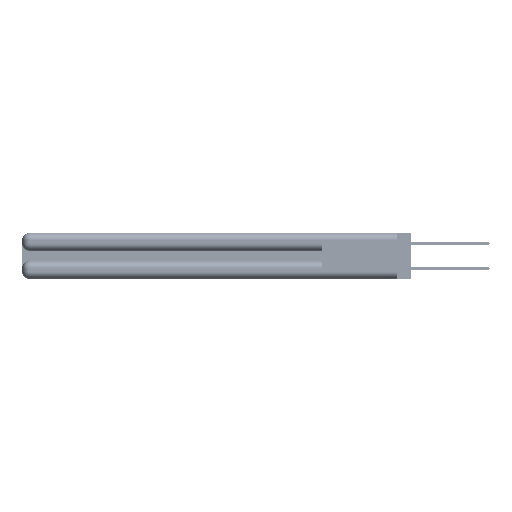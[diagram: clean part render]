
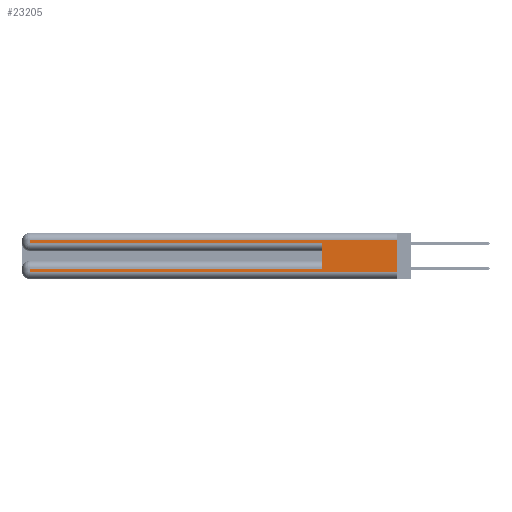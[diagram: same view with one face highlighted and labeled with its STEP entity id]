
A CAD part, left-side view. The second image highlights one B-rep face of the part: STEP entity #23205.
In plain terms, the highlighted planar face has unit normal (-1, 0, 0).
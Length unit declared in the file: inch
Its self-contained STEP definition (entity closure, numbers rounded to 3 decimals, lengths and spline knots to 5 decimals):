
#9 = VERTEX_POINT ( 'NONE', #21509 ) ;
#2199 = CARTESIAN_POINT ( 'NONE',  ( 0., 0., 0.37 ) ) ;
#2892 = FACE_OUTER_BOUND ( 'NONE', #34829, .T. ) ;
#3114 = DIRECTION ( 'NONE',  ( 0., 0., -1. ) ) ;
#3117 = ORIENTED_EDGE ( 'NONE', *, *, #11451, .F. ) ;
#3210 = VECTOR ( 'NONE', #3114, 39.37008 ) ;
#3261 = CARTESIAN_POINT ( 'NONE',  ( 0., 0., 0.31 ) ) ;
#3959 = ORIENTED_EDGE ( 'NONE', *, *, #20435, .T. ) ;
#4152 = LINE ( 'NONE', #50449, #15245 ) ;
#6395 = DIRECTION ( 'NONE',  ( 1., 0., 0. ) ) ;
#7473 = CARTESIAN_POINT ( 'NONE',  ( 0., 0.6, 0.145 ) ) ;
#10187 = VERTEX_POINT ( 'NONE', #29964 ) ;
#10823 = EDGE_CURVE ( 'NONE', #18976, #20659, #49497, .T. ) ;
#11451 = EDGE_CURVE ( 'NONE', #9, #26442, #22046, .T. ) ;
#12431 = VERTEX_POINT ( 'NONE', #44714 ) ;
#13711 = DIRECTION ( 'NONE',  ( 0., -1., 0. ) ) ;
#14200 = LINE ( 'NONE', #7473, #46127 ) ;
#15245 = VECTOR ( 'NONE', #33904, 39.37008 ) ;
#15658 = DIRECTION ( 'NONE',  ( 0., 1., 0. ) ) ;
#16292 = VECTOR ( 'NONE', #13711, 39.37008 ) ;
#16516 = CARTESIAN_POINT ( 'NONE',  ( 0., 0., 0.06 ) ) ;
#16888 = LINE ( 'NONE', #3261, #36416 ) ;
#17941 = LINE ( 'NONE', #16516, #19246 ) ;
#18580 = CARTESIAN_POINT ( 'NONE',  ( 0., 2.94, 0.37 ) ) ;
#18976 = VERTEX_POINT ( 'NONE', #26722 ) ;
#19246 = VECTOR ( 'NONE', #45658, 39.37008 ) ;
#19989 = ORIENTED_EDGE ( 'NONE', *, *, #34100, .T. ) ;
#20230 = EDGE_CURVE ( 'NONE', #10187, #45764, #34489, .T. ) ;
#20435 = EDGE_CURVE ( 'NONE', #37796, #18976, #37724, .T. ) ;
#20565 = ORIENTED_EDGE ( 'NONE', *, *, #44088, .T. ) ;
#20659 = VERTEX_POINT ( 'NONE', #21089 ) ;
#20756 = VECTOR ( 'NONE', #30204, 39.37008 ) ;
#21089 = CARTESIAN_POINT ( 'NONE',  ( 0., 0.6, 0.285 ) ) ;
#21509 = CARTESIAN_POINT ( 'NONE',  ( 0., 0., 0.31 ) ) ;
#22046 = LINE ( 'NONE', #50926, #20756 ) ;
#23205 = ADVANCED_FACE ( 'NONE', ( #2892 ), #52041, .F. ) ;
#24323 = EDGE_CURVE ( 'NONE', #12431, #10187, #4152, .T. ) ;
#25659 = CARTESIAN_POINT ( 'NONE',  ( 0., 2.94, 0.31 ) ) ;
#25860 = ORIENTED_EDGE ( 'NONE', *, *, #26623, .F. ) ;
#26442 = VERTEX_POINT ( 'NONE', #43898 ) ;
#26623 = EDGE_CURVE ( 'NONE', #12431, #20659, #14200, .T. ) ;
#26722 = CARTESIAN_POINT ( 'NONE',  ( 0., 2.94, 0.285 ) ) ;
#26766 = DIRECTION ( 'NONE',  ( 0., 0., -1. ) ) ;
#29470 = CARTESIAN_POINT ( 'NONE',  ( 0., 2.94, 0.06 ) ) ;
#29964 = CARTESIAN_POINT ( 'NONE',  ( 0., 2.94, 0.085 ) ) ;
#30204 = DIRECTION ( 'NONE',  ( 0., 0., -1. ) ) ;
#32487 = ORIENTED_EDGE ( 'NONE', *, *, #20230, .T. ) ;
#33904 = DIRECTION ( 'NONE',  ( 0., 1., 0. ) ) ;
#34100 = EDGE_CURVE ( 'NONE', #45764, #26442, #17941, .T. ) ;
#34242 = AXIS2_PLACEMENT_3D ( 'NONE', #2199, #6395, #35518 ) ;
#34444 = CARTESIAN_POINT ( 'NONE',  ( 0., 0., 0.285 ) ) ;
#34489 = LINE ( 'NONE', #18580, #44276 ) ;
#34829 = EDGE_LOOP ( 'NONE', ( #3117, #20565, #3959, #35669, #25860, #35206, #32487, #19989 ) ) ;
#35206 = ORIENTED_EDGE ( 'NONE', *, *, #24323, .T. ) ;
#35518 = DIRECTION ( 'NONE',  ( 0., 0., -1. ) ) ;
#35669 = ORIENTED_EDGE ( 'NONE', *, *, #10823, .T. ) ;
#36416 = VECTOR ( 'NONE', #15658, 39.37008 ) ;
#37724 = LINE ( 'NONE', #40421, #3210 ) ;
#37796 = VERTEX_POINT ( 'NONE', #25659 ) ;
#40421 = CARTESIAN_POINT ( 'NONE',  ( 0., 2.94, 0.37 ) ) ;
#43898 = CARTESIAN_POINT ( 'NONE',  ( 0., 0., 0.06 ) ) ;
#44088 = EDGE_CURVE ( 'NONE', #9, #37796, #16888, .T. ) ;
#44276 = VECTOR ( 'NONE', #26766, 39.37008 ) ;
#44714 = CARTESIAN_POINT ( 'NONE',  ( 0., 0.6, 0.085 ) ) ;
#45658 = DIRECTION ( 'NONE',  ( 0., -1., 0. ) ) ;
#45764 = VERTEX_POINT ( 'NONE', #29470 ) ;
#46127 = VECTOR ( 'NONE', #49131, 39.37008 ) ;
#49131 = DIRECTION ( 'NONE',  ( 0., 0., 1. ) ) ;
#49497 = LINE ( 'NONE', #34444, #16292 ) ;
#50449 = CARTESIAN_POINT ( 'NONE',  ( 0., 0., 0.085 ) ) ;
#50926 = CARTESIAN_POINT ( 'NONE',  ( 0., 0., 0.37 ) ) ;
#52041 = PLANE ( 'NONE',  #34242 ) ;
